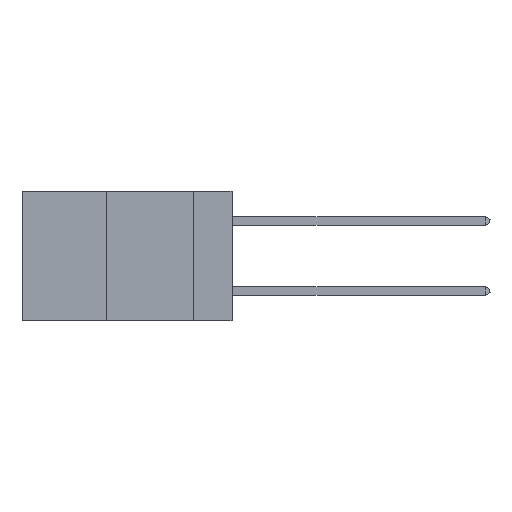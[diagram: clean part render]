
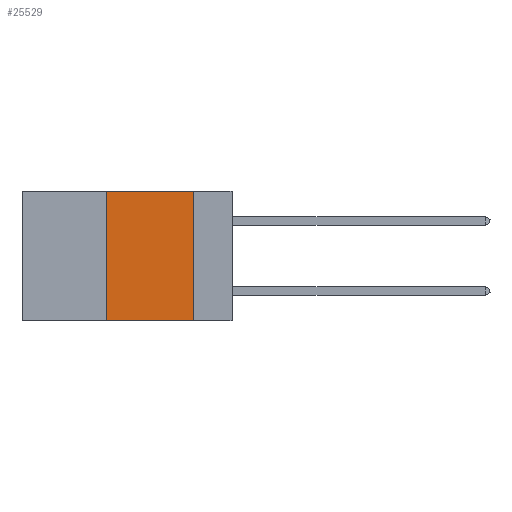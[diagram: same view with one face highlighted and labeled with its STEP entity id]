
A CAD part, left-side view. The second image highlights one B-rep face of the part: STEP entity #25529.
In plain terms, the highlighted planar face has unit normal (-1, 0, 0).
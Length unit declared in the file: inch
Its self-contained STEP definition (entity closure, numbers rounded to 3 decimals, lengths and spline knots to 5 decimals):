
#148 = DIRECTION ( 'NONE',  ( 0., 0., -1. ) ) ;
#825 = VERTEX_POINT ( 'NONE', #32802 ) ;
#829 = ORIENTED_EDGE ( 'NONE', *, *, #14749, .T. ) ;
#3156 = CARTESIAN_POINT ( 'NONE',  ( 0., 0.6, 0. ) ) ;
#8227 = CARTESIAN_POINT ( 'NONE',  ( 0., 0.36, -0.37 ) ) ;
#8342 = FACE_OUTER_BOUND ( 'NONE', #31450, .T. ) ;
#8709 = VERTEX_POINT ( 'NONE', #34871 ) ;
#9016 = CARTESIAN_POINT ( 'NONE',  ( 0., 0.36, 0. ) ) ;
#9098 = AXIS2_PLACEMENT_3D ( 'NONE', #3156, #16661, #148 ) ;
#12927 = DIRECTION ( 'NONE',  ( 0., -1., 0. ) ) ;
#14749 = EDGE_CURVE ( 'NONE', #26740, #8709, #34081, .T. ) ;
#15147 = CARTESIAN_POINT ( 'NONE',  ( 0., 0.11, 0. ) ) ;
#15591 = CARTESIAN_POINT ( 'NONE',  ( 0., 0.6, -0.37 ) ) ;
#16661 = DIRECTION ( 'NONE',  ( 1., 0., 0. ) ) ;
#18083 = ORIENTED_EDGE ( 'NONE', *, *, #19648, .F. ) ;
#19103 = LINE ( 'NONE', #9016, #28985 ) ;
#19648 = EDGE_CURVE ( 'NONE', #825, #8709, #22124, .T. ) ;
#20526 = VERTEX_POINT ( 'NONE', #25237 ) ;
#20879 = EDGE_CURVE ( 'NONE', #20526, #825, #29774, .T. ) ;
#22124 = LINE ( 'NONE', #15147, #27255 ) ;
#22369 = PLANE ( 'NONE',  #9098 ) ;
#22752 = DIRECTION ( 'NONE',  ( 0., 0., 1. ) ) ;
#25237 = CARTESIAN_POINT ( 'NONE',  ( 0., 0.36, 0. ) ) ;
#25473 = VECTOR ( 'NONE', #12927, 39.37008 ) ;
#25529 = ADVANCED_FACE ( 'NONE', ( #8342 ), #22369, .F. ) ;
#26020 = DIRECTION ( 'NONE',  ( 0., 0., -1. ) ) ;
#26740 = VERTEX_POINT ( 'NONE', #8227 ) ;
#26743 = VECTOR ( 'NONE', #32012, 39.37008 ) ;
#27255 = VECTOR ( 'NONE', #26020, 39.37008 ) ;
#27591 = EDGE_CURVE ( 'NONE', #26740, #20526, #19103, .T. ) ;
#28985 = VECTOR ( 'NONE', #22752, 39.37008 ) ;
#29774 = LINE ( 'NONE', #32427, #25473 ) ;
#31435 = ORIENTED_EDGE ( 'NONE', *, *, #27591, .F. ) ;
#31450 = EDGE_LOOP ( 'NONE', ( #18083, #35129, #31435, #829 ) ) ;
#32012 = DIRECTION ( 'NONE',  ( 0., -1., 0. ) ) ;
#32427 = CARTESIAN_POINT ( 'NONE',  ( 0., 0.6, 0. ) ) ;
#32802 = CARTESIAN_POINT ( 'NONE',  ( 0., 0.11, 0. ) ) ;
#34081 = LINE ( 'NONE', #15591, #26743 ) ;
#34871 = CARTESIAN_POINT ( 'NONE',  ( 0., 0.11, -0.37 ) ) ;
#35129 = ORIENTED_EDGE ( 'NONE', *, *, #20879, .F. ) ;
